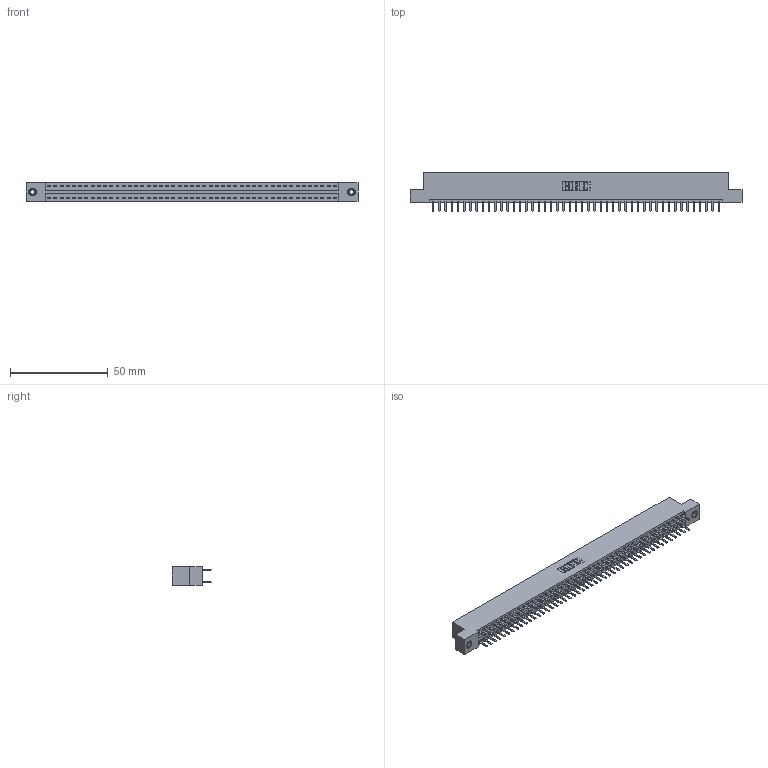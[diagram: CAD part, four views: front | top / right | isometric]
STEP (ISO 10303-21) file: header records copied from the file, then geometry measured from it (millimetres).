
FILE_DESCRIPTION (( 'STEP AP203' ), '1' );
FILE_NAME ('396-094-520-208.STEP', '2018-09-12T11:58:59', ( '' ), ( '' ), 'SwSTEP 2.0', 'SolidWorks 2016', '' );
FILE_SCHEMA (( 'CONFIG_CONTROL_DESIGN' ));
Length unit declared in the file: inch
Products named in the file (4): 346 Part_Flush Mounting Lugs - 0.156 Dia-TI; 345-292-001_345-293-120; 345-250-001_345-250-003-102; 396-094-520-208
Assembly tree (97 placements, depth 2):
  396-094-520-208
    346 Part_Flush Mounting Lugs - 0.156 Dia-TI
    345-292-001_345-293-120  x94
    345-250-001_345-250-003-102  x2
Bounding box: 169.8 x 20.02 x 9.4 mm (x, y, z)
Volume: 16548.5 mm3; surface area: 22748.8 mm2
Topology: 97 solids, 97 shells, 5446 faces, 15787 edges, 10266 vertices
Faces by surface type: plane 3586, cylinder 1844, cone 12, torus 4
Entity records: 31300 total; most frequent: CARTESIAN_POINT 5147, ORIENTED_EDGE 5062, DIRECTION 4601, EDGE_CURVE 2531, LINE 2187, VECTOR 2187, VERTEX_POINT 1680, AXIS2_PLACEMENT_3D 1207
